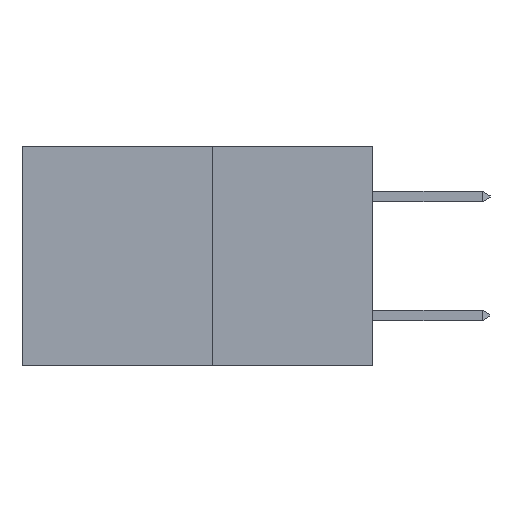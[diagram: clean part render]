
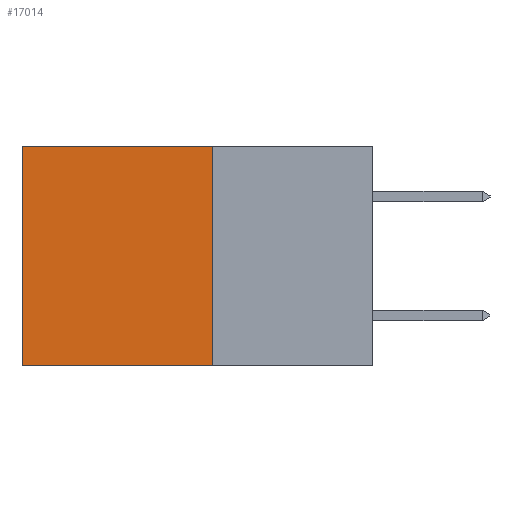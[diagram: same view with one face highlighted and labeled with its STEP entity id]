
A CAD part, left-side view. The second image highlights one B-rep face of the part: STEP entity #17014.
In plain terms, the highlighted planar face has unit normal (-1, 0, 0).
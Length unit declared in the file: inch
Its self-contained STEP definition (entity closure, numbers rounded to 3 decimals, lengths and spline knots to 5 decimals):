
#674 = CARTESIAN_POINT ( 'NONE',  ( 0.277, 0.27, -0.37 ) ) ;
#1207 = VECTOR ( 'NONE', #3828, 39.37008 ) ;
#2466 = DIRECTION ( 'NONE',  ( 1., 0., 0. ) ) ;
#2720 = ORIENTED_EDGE ( 'NONE', *, *, #9152, .T. ) ;
#3337 = DIRECTION ( 'NONE',  ( 0., 0., -1. ) ) ;
#3651 = CARTESIAN_POINT ( 'NONE',  ( 0.277, 0.27, 0. ) ) ;
#3828 = DIRECTION ( 'NONE',  ( 0., 1., 0. ) ) ;
#4009 = LINE ( 'NONE', #8365, #21323 ) ;
#4924 = FACE_OUTER_BOUND ( 'NONE', #13244, .T. ) ;
#5228 = CARTESIAN_POINT ( 'NONE',  ( 0.277, 0.27, -0.37 ) ) ;
#5484 = AXIS2_PLACEMENT_3D ( 'NONE', #674, #2466, #14382 ) ;
#6705 = CARTESIAN_POINT ( 'NONE',  ( 0.277, 0.59, 0. ) ) ;
#6960 = DIRECTION ( 'NONE',  ( 0., 1., 0. ) ) ;
#7292 = DIRECTION ( 'NONE',  ( 0., 0., -1. ) ) ;
#7441 = VECTOR ( 'NONE', #7292, 39.37008 ) ;
#7907 = CARTESIAN_POINT ( 'NONE',  ( 0.277, 0.59, -0.37 ) ) ;
#7961 = VECTOR ( 'NONE', #6960, 39.37008 ) ;
#8010 = LINE ( 'NONE', #3651, #1207 ) ;
#8355 = ORIENTED_EDGE ( 'NONE', *, *, #12532, .F. ) ;
#8365 = CARTESIAN_POINT ( 'NONE',  ( 0.277, 0.27, -0.37 ) ) ;
#9152 = EDGE_CURVE ( 'NONE', #10381, #21025, #8010, .T. ) ;
#10381 = VERTEX_POINT ( 'NONE', #12373 ) ;
#10992 = PLANE ( 'NONE',  #5484 ) ;
#11622 = EDGE_CURVE ( 'NONE', #21025, #18473, #12985, .T. ) ;
#11715 = ORIENTED_EDGE ( 'NONE', *, *, #11622, .T. ) ;
#12373 = CARTESIAN_POINT ( 'NONE',  ( 0.277, 0.27, 0. ) ) ;
#12396 = CARTESIAN_POINT ( 'NONE',  ( 0.277, 0.59, -0.37 ) ) ;
#12532 = EDGE_CURVE ( 'NONE', #13601, #18473, #12965, .T. ) ;
#12965 = LINE ( 'NONE', #5228, #7961 ) ;
#12985 = LINE ( 'NONE', #12396, #7441 ) ;
#13244 = EDGE_LOOP ( 'NONE', ( #11715, #8355, #18991, #2720 ) ) ;
#13601 = VERTEX_POINT ( 'NONE', #18200 ) ;
#14382 = DIRECTION ( 'NONE',  ( 0., 0., -1. ) ) ;
#17014 = ADVANCED_FACE ( 'NONE', ( #4924 ), #10992, .F. ) ;
#17966 = EDGE_CURVE ( 'NONE', #10381, #13601, #4009, .T. ) ;
#18200 = CARTESIAN_POINT ( 'NONE',  ( 0.277, 0.27, -0.37 ) ) ;
#18473 = VERTEX_POINT ( 'NONE', #7907 ) ;
#18991 = ORIENTED_EDGE ( 'NONE', *, *, #17966, .F. ) ;
#21025 = VERTEX_POINT ( 'NONE', #6705 ) ;
#21323 = VECTOR ( 'NONE', #3337, 39.37008 ) ;
